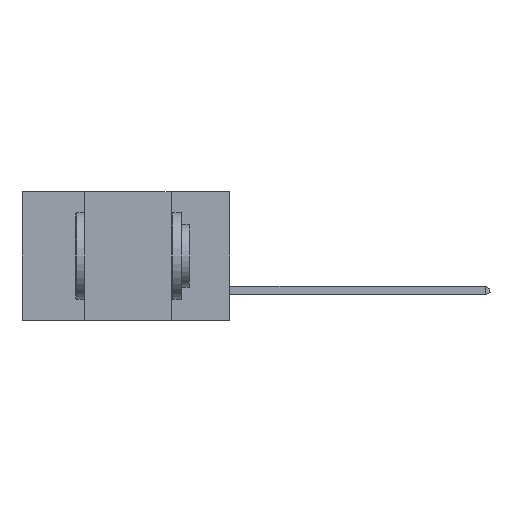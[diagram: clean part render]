
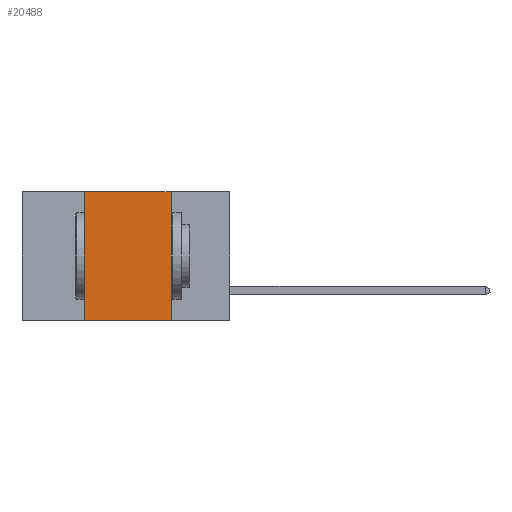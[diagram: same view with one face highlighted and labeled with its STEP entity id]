
A CAD part, left-side view. The second image highlights one B-rep face of the part: STEP entity #20488.
In plain terms, the highlighted planar face has unit normal (-1, 0, 0).
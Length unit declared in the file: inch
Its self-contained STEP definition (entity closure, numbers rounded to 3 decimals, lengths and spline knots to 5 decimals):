
#92 = EDGE_CURVE ( 'NONE', #1842, #12527, #5886, .T. ) ;
#123 = DIRECTION ( 'NONE',  ( 0., 0., -1. ) ) ;
#552 = LINE ( 'NONE', #20592, #15115 ) ;
#737 = VECTOR ( 'NONE', #24630, 39.37008 ) ;
#1630 = DIRECTION ( 'NONE',  ( 0., -1., 0. ) ) ;
#1842 = VERTEX_POINT ( 'NONE', #17092 ) ;
#1901 = EDGE_CURVE ( 'NONE', #14152, #12527, #10294, .T. ) ;
#2444 = CARTESIAN_POINT ( 'NONE',  ( 0., 0.17, 0. ) ) ;
#3337 = DIRECTION ( 'NONE',  ( 1., 0., 0. ) ) ;
#4569 = DIRECTION ( 'NONE',  ( 0., 0., -1. ) ) ;
#5886 = LINE ( 'NONE', #2444, #16503 ) ;
#6298 = ORIENTED_EDGE ( 'NONE', *, *, #92, .F. ) ;
#8603 = CARTESIAN_POINT ( 'NONE',  ( 0., 0.17, -0.37 ) ) ;
#9030 = EDGE_CURVE ( 'NONE', #14152, #15957, #552, .T. ) ;
#9405 = VECTOR ( 'NONE', #1630, 39.37008 ) ;
#9425 = EDGE_LOOP ( 'NONE', ( #6298, #13984, #13506, #22736 ) ) ;
#10294 = LINE ( 'NONE', #22711, #9405 ) ;
#10849 = CARTESIAN_POINT ( 'NONE',  ( 0., 0.42, -0.37 ) ) ;
#10983 = LINE ( 'NONE', #20300, #737 ) ;
#12527 = VERTEX_POINT ( 'NONE', #8603 ) ;
#12939 = DIRECTION ( 'NONE',  ( 0., 0., 1. ) ) ;
#13301 = CARTESIAN_POINT ( 'NONE',  ( 0., 0.6, 0. ) ) ;
#13506 = ORIENTED_EDGE ( 'NONE', *, *, #9030, .F. ) ;
#13984 = ORIENTED_EDGE ( 'NONE', *, *, #15772, .F. ) ;
#14152 = VERTEX_POINT ( 'NONE', #10849 ) ;
#14495 = CARTESIAN_POINT ( 'NONE',  ( 0., 0.42, 0. ) ) ;
#15115 = VECTOR ( 'NONE', #12939, 39.37008 ) ;
#15772 = EDGE_CURVE ( 'NONE', #15957, #1842, #10983, .T. ) ;
#15957 = VERTEX_POINT ( 'NONE', #14495 ) ;
#16503 = VECTOR ( 'NONE', #4569, 39.37008 ) ;
#16664 = FACE_OUTER_BOUND ( 'NONE', #9425, .T. ) ;
#17092 = CARTESIAN_POINT ( 'NONE',  ( 0., 0.17, 0. ) ) ;
#20300 = CARTESIAN_POINT ( 'NONE',  ( 0., 0.6, 0. ) ) ;
#20488 = ADVANCED_FACE ( 'NONE', ( #16664 ), #24429, .F. ) ;
#20592 = CARTESIAN_POINT ( 'NONE',  ( 0., 0.42, 0. ) ) ;
#22711 = CARTESIAN_POINT ( 'NONE',  ( 0., 0.6, -0.37 ) ) ;
#22736 = ORIENTED_EDGE ( 'NONE', *, *, #1901, .T. ) ;
#23644 = AXIS2_PLACEMENT_3D ( 'NONE', #13301, #3337, #123 ) ;
#24429 = PLANE ( 'NONE',  #23644 ) ;
#24630 = DIRECTION ( 'NONE',  ( 0., -1., 0. ) ) ;
